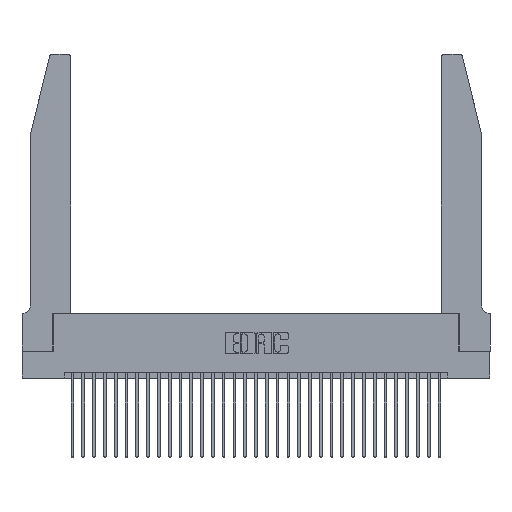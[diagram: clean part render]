
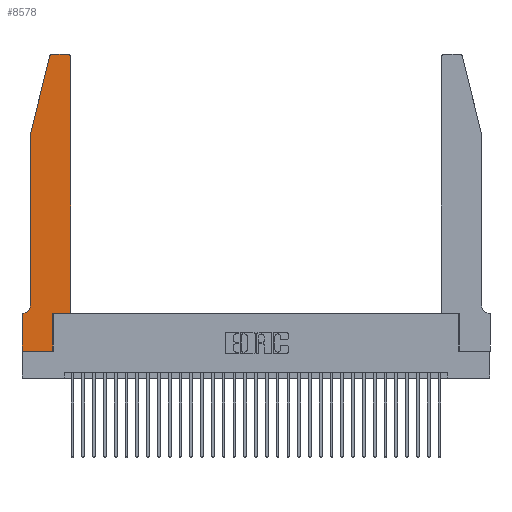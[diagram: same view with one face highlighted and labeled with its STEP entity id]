
A CAD part, top view. The second image highlights one B-rep face of the part: STEP entity #8578.
In plain terms, the highlighted planar face has unit normal (0, 0, 1).
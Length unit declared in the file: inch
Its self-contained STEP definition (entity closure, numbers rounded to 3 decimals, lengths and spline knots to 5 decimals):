
#192 = VECTOR ( 'NONE', #14699, 39.37008 ) ;
#197 = VERTEX_POINT ( 'NONE', #1971 ) ;
#265 = ORIENTED_EDGE ( 'NONE', *, *, #27216, .T. ) ;
#394 = ORIENTED_EDGE ( 'NONE', *, *, #12575, .T. ) ;
#1292 = DIRECTION ( 'NONE',  ( -0.239, -0.971, 0. ) ) ;
#1971 = CARTESIAN_POINT ( 'NONE',  ( 0.4205, 2.75, 0.37 ) ) ;
#2623 = VERTEX_POINT ( 'NONE', #4574 ) ;
#3056 = LINE ( 'NONE', #19361, #16005 ) ;
#3524 = ORIENTED_EDGE ( 'NONE', *, *, #10339, .T. ) ;
#3733 = ORIENTED_EDGE ( 'NONE', *, *, #18767, .T. ) ;
#3865 = VECTOR ( 'NONE', #26477, 39.37008 ) ;
#4574 = CARTESIAN_POINT ( 'NONE',  ( 0.2865, 0., 0.37 ) ) ;
#4599 = LINE ( 'NONE', #28196, #30989 ) ;
#5566 = AXIS2_PLACEMENT_3D ( 'NONE', #22404, #7019, #24960 ) ;
#5783 = ORIENTED_EDGE ( 'NONE', *, *, #7692, .T. ) ;
#6936 = EDGE_CURVE ( 'NONE', #12745, #25979, #15267, .T. ) ;
#7019 = DIRECTION ( 'NONE',  ( 0., 0., 1. ) ) ;
#7187 = LINE ( 'NONE', #24881, #192 ) ;
#7233 = ORIENTED_EDGE ( 'NONE', *, *, #29853, .T. ) ;
#7684 = PLANE ( 'NONE',  #26021 ) ;
#7692 = EDGE_CURVE ( 'NONE', #22154, #32050, #7187, .T. ) ;
#7942 = CARTESIAN_POINT ( 'NONE',  ( 0., 0.35, 0.37 ) ) ;
#8264 = EDGE_CURVE ( 'NONE', #16018, #12745, #3056, .T. ) ;
#8458 = VERTEX_POINT ( 'NONE', #14875 ) ;
#8578 = ADVANCED_FACE ( 'NONE', ( #28345 ), #7684, .T. ) ;
#9163 = CARTESIAN_POINT ( 'NONE',  ( 0.25487, 2.72718, 0.37 ) ) ;
#9430 = ORIENTED_EDGE ( 'NONE', *, *, #26064, .T. ) ;
#9786 = CARTESIAN_POINT ( 'NONE',  ( 0., 0., 0.37 ) ) ;
#9940 = VERTEX_POINT ( 'NONE', #15837 ) ;
#10302 = DIRECTION ( 'NONE',  ( 0., 0., 1. ) ) ;
#10339 = EDGE_CURVE ( 'NONE', #13735, #8458, #4599, .T. ) ;
#11621 = CARTESIAN_POINT ( 'NONE',  ( 0.4505, 2.72, 0.37 ) ) ;
#12185 = DIRECTION ( 'NONE',  ( 0., 0., -1. ) ) ;
#12460 = VECTOR ( 'NONE', #15386, 39.37008 ) ;
#12575 = EDGE_CURVE ( 'NONE', #16830, #13735, #31066, .T. ) ;
#12745 = VERTEX_POINT ( 'NONE', #32051 ) ;
#13105 = CARTESIAN_POINT ( 'NONE',  ( 0.284, 2.72, 0.37 ) ) ;
#13735 = VERTEX_POINT ( 'NONE', #7942 ) ;
#14173 = LINE ( 'NONE', #9786, #30090 ) ;
#14312 = CARTESIAN_POINT ( 'NONE',  ( 0.2605, 2.75, 0.37 ) ) ;
#14358 = EDGE_LOOP ( 'NONE', ( #265, #9430, #28037, #30550, #7233, #394, #3524, #26753, #3733, #32738, #5783, #27562 ) ) ;
#14488 = VECTOR ( 'NONE', #16530, 39.37008 ) ;
#14699 = DIRECTION ( 'NONE',  ( 0., 1., 0. ) ) ;
#14875 = CARTESIAN_POINT ( 'NONE',  ( 0., 0., 0.37 ) ) ;
#15221 = CARTESIAN_POINT ( 'NONE',  ( 0.0755, 0.42, 0.37 ) ) ;
#15230 = VECTOR ( 'NONE', #18786, 39.37008 ) ;
#15267 = LINE ( 'NONE', #26694, #14488 ) ;
#15334 = CIRCLE ( 'NONE', #20997, 0.03 ) ;
#15386 = DIRECTION ( 'NONE',  ( 0., 1., 0. ) ) ;
#15397 = CARTESIAN_POINT ( 'NONE',  ( 0.4505, 0.35, 0.37 ) ) ;
#15688 = DIRECTION ( 'NONE',  ( 1., 0., 0. ) ) ;
#15837 = CARTESIAN_POINT ( 'NONE',  ( 0.284, 2.75, 0.37 ) ) ;
#16005 = VECTOR ( 'NONE', #1292, 39.37008 ) ;
#16018 = VERTEX_POINT ( 'NONE', #9163 ) ;
#16065 = AXIS2_PLACEMENT_3D ( 'NONE', #27485, #12185, #30005 ) ;
#16207 = CARTESIAN_POINT ( 'NONE',  ( 0.4505, 0.35, 0.37 ) ) ;
#16530 = DIRECTION ( 'NONE',  ( 0., -1., 0. ) ) ;
#16830 = VERTEX_POINT ( 'NONE', #27423 ) ;
#18059 = DIRECTION ( 'NONE',  ( 0., -1., 0. ) ) ;
#18767 = EDGE_CURVE ( 'NONE', #2623, #22438, #19267, .T. ) ;
#18786 = DIRECTION ( 'NONE',  ( 1., 0., 0. ) ) ;
#19237 = CIRCLE ( 'NONE', #5566, 0.03 ) ;
#19267 = LINE ( 'NONE', #28117, #12460 ) ;
#19361 = CARTESIAN_POINT ( 'NONE',  ( 0.0755, 2., 0.37 ) ) ;
#20310 = CIRCLE ( 'NONE', #16065, 0.07 ) ;
#20997 = AXIS2_PLACEMENT_3D ( 'NONE', #13105, #30877, #15688 ) ;
#21971 = CARTESIAN_POINT ( 'NONE',  ( 0.2865, 0.35, 0.37 ) ) ;
#22041 = LINE ( 'NONE', #16207, #15230 ) ;
#22154 = VERTEX_POINT ( 'NONE', #15397 ) ;
#22404 = CARTESIAN_POINT ( 'NONE',  ( 0.4205, 2.72, 0.37 ) ) ;
#22438 = VERTEX_POINT ( 'NONE', #21971 ) ;
#22934 = VECTOR ( 'NONE', #29570, 39.37008 ) ;
#23043 = CARTESIAN_POINT ( 'NONE',  ( 0., 0.35, 0.37 ) ) ;
#23926 = CARTESIAN_POINT ( 'NONE',  ( 0.0755, 0.35, 0.37 ) ) ;
#24881 = CARTESIAN_POINT ( 'NONE',  ( 0.4505, 0.35, 0.37 ) ) ;
#24960 = DIRECTION ( 'NONE',  ( 1., 0., 0. ) ) ;
#25842 = EDGE_CURVE ( 'NONE', #8458, #2623, #14173, .T. ) ;
#25979 = VERTEX_POINT ( 'NONE', #15221 ) ;
#26021 = AXIS2_PLACEMENT_3D ( 'NONE', #23043, #10302, #28157 ) ;
#26064 = EDGE_CURVE ( 'NONE', #9940, #16018, #15334, .T. ) ;
#26477 = DIRECTION ( 'NONE',  ( -1., 0., 0. ) ) ;
#26694 = CARTESIAN_POINT ( 'NONE',  ( 0.0755, 2., 0.37 ) ) ;
#26753 = ORIENTED_EDGE ( 'NONE', *, *, #25842, .T. ) ;
#27216 = EDGE_CURVE ( 'NONE', #197, #9940, #30427, .T. ) ;
#27423 = CARTESIAN_POINT ( 'NONE',  ( 0.0055, 0.35, 0.37 ) ) ;
#27485 = CARTESIAN_POINT ( 'NONE',  ( 0.0055, 0.42, 0.37 ) ) ;
#27562 = ORIENTED_EDGE ( 'NONE', *, *, #28469, .T. ) ;
#27635 = DIRECTION ( 'NONE',  ( 1., 0., 0. ) ) ;
#28037 = ORIENTED_EDGE ( 'NONE', *, *, #8264, .T. ) ;
#28117 = CARTESIAN_POINT ( 'NONE',  ( 0.2865, 0.35, 0.37 ) ) ;
#28157 = DIRECTION ( 'NONE',  ( 1., 0., 0. ) ) ;
#28196 = CARTESIAN_POINT ( 'NONE',  ( 0., 0., 0.37 ) ) ;
#28345 = FACE_OUTER_BOUND ( 'NONE', #14358, .T. ) ;
#28469 = EDGE_CURVE ( 'NONE', #32050, #197, #19237, .T. ) ;
#29570 = DIRECTION ( 'NONE',  ( -1., 0., 0. ) ) ;
#29853 = EDGE_CURVE ( 'NONE', #25979, #16830, #20310, .T. ) ;
#30005 = DIRECTION ( 'NONE',  ( -1., 0., 0. ) ) ;
#30090 = VECTOR ( 'NONE', #27635, 39.37008 ) ;
#30427 = LINE ( 'NONE', #14312, #22934 ) ;
#30550 = ORIENTED_EDGE ( 'NONE', *, *, #6936, .T. ) ;
#30877 = DIRECTION ( 'NONE',  ( 0., 0., 1. ) ) ;
#30989 = VECTOR ( 'NONE', #18059, 39.37008 ) ;
#31066 = LINE ( 'NONE', #23926, #3865 ) ;
#31956 = EDGE_CURVE ( 'NONE', #22438, #22154, #22041, .T. ) ;
#32050 = VERTEX_POINT ( 'NONE', #11621 ) ;
#32051 = CARTESIAN_POINT ( 'NONE',  ( 0.0755, 2., 0.37 ) ) ;
#32738 = ORIENTED_EDGE ( 'NONE', *, *, #31956, .T. ) ;
